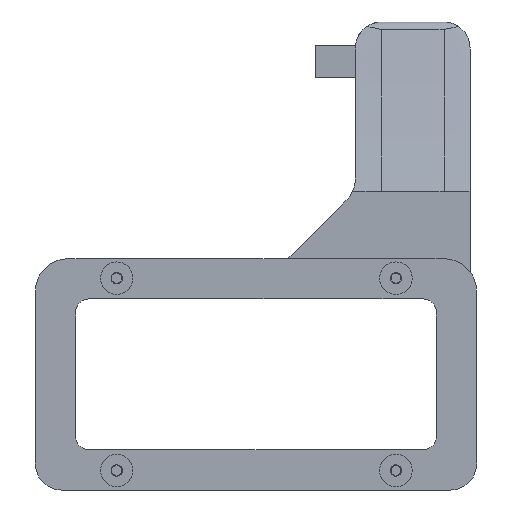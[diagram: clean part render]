
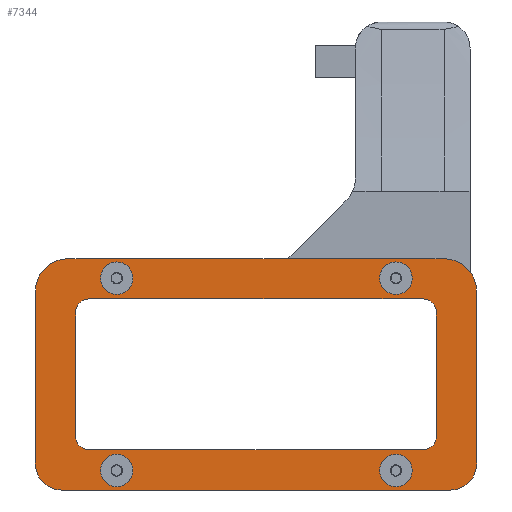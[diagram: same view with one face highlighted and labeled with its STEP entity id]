
A CAD part, front view. The second image highlights one B-rep face of the part: STEP entity #7344.
In plain terms, the highlighted planar face has unit normal (0, -1, 0).
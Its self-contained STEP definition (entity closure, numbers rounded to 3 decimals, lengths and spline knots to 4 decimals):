
#148=LINE($,#29468,#426);
#155=LINE($,#29518,#433);
#163=LINE($,#29570,#441);
#168=LINE($,#29579,#446);
#172=LINE($,#29596,#450);
#175=LINE($,#29603,#453);
#176=LINE($,#29606,#454);
#177=LINE($,#29607,#455);
#178=LINE($,#29613,#456);
#179=LINE($,#29615,#457);
#180=LINE($,#29617,#458);
#181=LINE($,#29621,#459);
#426=VECTOR($,#8607,2.6586);
#433=VECTOR($,#8652,1.9192);
#441=VECTOR($,#8702,5.1467);
#446=VECTOR($,#8709,5.986);
#450=VECTOR($,#8725,0.1144);
#453=VECTOR($,#8732,2.6586);
#454=VECTOR($,#8735,2.704);
#455=VECTOR($,#8736,2.9676);
#456=VECTOR($,#8741,2.648);
#457=VECTOR($,#8742,0.1144);
#458=VECTOR($,#8743,2.3843);
#459=VECTOR($,#8746,1.9192);
#653=FACE_BOUND($,#1912,.T.);
#654=FACE_BOUND($,#1913,.T.);
#655=FACE_BOUND($,#1914,.T.);
#656=FACE_BOUND($,#1915,.T.);
#657=FACE_BOUND($,#1916,.T.);
#757=PLANE($,#7790);
#1577=FACE_OUTER_BOUND($,#1911,.T.);
#1911=EDGE_LOOP($,(#6174,#6175,#6176,#6177,#6178,#6179,#6180,#6181,#6182,
#6183));
#1912=EDGE_LOOP($,(#6184));
#1913=EDGE_LOOP($,(#6185));
#1914=EDGE_LOOP($,(#6186));
#1915=EDGE_LOOP($,(#6187));
#1916=EDGE_LOOP($,(#6188,#6189,#6190,#6191,#6192,#6193,#6194,#6195,#6196,
#6197));
#2178=CIRCLE($,#7741,0.5);
#2189=CIRCLE($,#7758,0.2);
#2190=CIRCLE($,#7760,0.2);
#2192=CIRCLE($,#7765,0.25);
#2195=CIRCLE($,#7770,0.25);
#2196=CIRCLE($,#7772,0.4);
#2205=CIRCLE($,#7791,0.4);
#2206=CIRCLE($,#7792,0.5);
#2207=CIRCLE($,#7793,0.25);
#2208=CIRCLE($,#7794,0.25);
#2209=CIRCLE($,#7795,0.2);
#2210=CIRCLE($,#7796,0.2);
#3079=VERTEX_POINT($,#29460);
#3080=VERTEX_POINT($,#29462);
#3081=VERTEX_POINT($,#29466);
#3094=VERTEX_POINT($,#29506);
#3095=VERTEX_POINT($,#29508);
#3096=VERTEX_POINT($,#29512);
#3097=VERTEX_POINT($,#29514);
#3099=VERTEX_POINT($,#29523);
#3102=VERTEX_POINT($,#29531);
#3103=VERTEX_POINT($,#29534);
#3114=VERTEX_POINT($,#29569);
#3117=VERTEX_POINT($,#29577);
#3123=VERTEX_POINT($,#29594);
#3124=VERTEX_POINT($,#29595);
#3125=VERTEX_POINT($,#29600);
#3126=VERTEX_POINT($,#29602);
#3127=VERTEX_POINT($,#29604);
#3128=VERTEX_POINT($,#29608);
#3129=VERTEX_POINT($,#29610);
#3130=VERTEX_POINT($,#29612);
#3131=VERTEX_POINT($,#29614);
#3132=VERTEX_POINT($,#29616);
#3133=VERTEX_POINT($,#29618);
#3134=VERTEX_POINT($,#29620);
#4165=EDGE_CURVE($,#3080,#3079,#2178,.T.);
#4168=EDGE_CURVE($,#3079,#3081,#148,.T.);
#4184=EDGE_CURVE($,#3094,#3095,#2189,.T.);
#4187=EDGE_CURVE($,#3096,#3097,#2190,.T.);
#4189=EDGE_CURVE($,#3094,#3097,#155,.T.);
#4191=EDGE_CURVE($,#3099,#3099,#2192,.T.);
#4194=EDGE_CURVE($,#3102,#3102,#2195,.T.);
#4196=EDGE_CURVE($,#3081,#3103,#2196,.T.);
#4209=EDGE_CURVE($,#3114,#3095,#163,.T.);
#4214=EDGE_CURVE($,#3103,#3117,#168,.T.);
#4221=EDGE_CURVE($,#3123,#3124,#172,.T.);
#4224=EDGE_CURVE($,#3117,#3125,#2205,.T.);
#4225=EDGE_CURVE($,#3125,#3126,#175,.T.);
#4226=EDGE_CURVE($,#3126,#3127,#2206,.T.);
#4227=EDGE_CURVE($,#3127,#3123,#176,.T.);
#4228=EDGE_CURVE($,#3124,#3080,#177,.T.);
#4229=EDGE_CURVE($,#3128,#3128,#2207,.T.);
#4230=EDGE_CURVE($,#3129,#3129,#2208,.T.);
#4231=EDGE_CURVE($,#3096,#3130,#178,.T.);
#4232=EDGE_CURVE($,#3130,#3131,#179,.T.);
#4233=EDGE_CURVE($,#3131,#3132,#180,.T.);
#4234=EDGE_CURVE($,#3133,#3132,#2209,.T.);
#4235=EDGE_CURVE($,#3133,#3134,#181,.T.);
#4236=EDGE_CURVE($,#3114,#3134,#2210,.T.);
#6174=ORIENTED_EDGE($,*,*,#4214,.T.);
#6175=ORIENTED_EDGE($,*,*,#4224,.T.);
#6176=ORIENTED_EDGE($,*,*,#4225,.T.);
#6177=ORIENTED_EDGE($,*,*,#4226,.T.);
#6178=ORIENTED_EDGE($,*,*,#4227,.T.);
#6179=ORIENTED_EDGE($,*,*,#4221,.T.);
#6180=ORIENTED_EDGE($,*,*,#4228,.T.);
#6181=ORIENTED_EDGE($,*,*,#4165,.T.);
#6182=ORIENTED_EDGE($,*,*,#4168,.T.);
#6183=ORIENTED_EDGE($,*,*,#4196,.T.);
#6184=ORIENTED_EDGE($,*,*,#4191,.T.);
#6185=ORIENTED_EDGE($,*,*,#4194,.T.);
#6186=ORIENTED_EDGE($,*,*,#4229,.T.);
#6187=ORIENTED_EDGE($,*,*,#4230,.T.);
#6188=ORIENTED_EDGE($,*,*,#4209,.T.);
#6189=ORIENTED_EDGE($,*,*,#4184,.F.);
#6190=ORIENTED_EDGE($,*,*,#4189,.T.);
#6191=ORIENTED_EDGE($,*,*,#4187,.F.);
#6192=ORIENTED_EDGE($,*,*,#4231,.T.);
#6193=ORIENTED_EDGE($,*,*,#4232,.T.);
#6194=ORIENTED_EDGE($,*,*,#4233,.T.);
#6195=ORIENTED_EDGE($,*,*,#4234,.F.);
#6196=ORIENTED_EDGE($,*,*,#4235,.T.);
#6197=ORIENTED_EDGE($,*,*,#4236,.F.);
#7344=ADVANCED_FACE($,(#1577,#653,#654,#655,#656,#657),#757,.T.);
#7741=AXIS2_PLACEMENT_3D($,#29463,#8601,#8602);
#7758=AXIS2_PLACEMENT_3D($,#29509,#8641,#8642);
#7760=AXIS2_PLACEMENT_3D($,#29515,#8647,#8648);
#7765=AXIS2_PLACEMENT_3D($,#29524,#8659,#8660);
#7770=AXIS2_PLACEMENT_3D($,#29532,#8669,#8670);
#7772=AXIS2_PLACEMENT_3D($,#29536,#8674,#8675);
#7790=AXIS2_PLACEMENT_3D($,#29599,#8728,#8729);
#7791=AXIS2_PLACEMENT_3D($,#29601,#8730,#8731);
#7792=AXIS2_PLACEMENT_3D($,#29605,#8733,#8734);
#7793=AXIS2_PLACEMENT_3D($,#29609,#8737,#8738);
#7794=AXIS2_PLACEMENT_3D($,#29611,#8739,#8740);
#7795=AXIS2_PLACEMENT_3D($,#29619,#8744,#8745);
#7796=AXIS2_PLACEMENT_3D($,#29622,#8747,#8748);
#8601=DIRECTION('center_axis',(0.,-1.,0.));
#8602=DIRECTION('ref_axis',(0.,0.,1.));
#8607=DIRECTION($,(0.,0.,-1.));
#8641=DIRECTION('center_axis',(0.,-1.,0.));
#8642=DIRECTION('ref_axis',(-0.707,0.,-0.707));
#8647=DIRECTION('center_axis',(0.,-1.,0.));
#8648=DIRECTION('ref_axis',(-0.707,0.,0.707));
#8652=DIRECTION($,(0.,0.,1.));
#8659=DIRECTION('center_axis',(0.,1.,0.));
#8660=DIRECTION('ref_axis',(0.,0.,-1.));
#8669=DIRECTION('center_axis',(0.,1.,0.));
#8670=DIRECTION('ref_axis',(0.,0.,-1.));
#8674=DIRECTION('center_axis',(0.,-1.,0.));
#8675=DIRECTION('ref_axis',(-1.,0.,0.));
#8702=DIRECTION($,(-1.,0.,0.));
#8709=DIRECTION($,(1.,0.,0.));
#8725=DIRECTION($,(-1.,0.,0.));
#8728=DIRECTION('center_axis',(0.,-1.,0.));
#8729=DIRECTION('ref_axis',(1.,0.,0.));
#8730=DIRECTION('center_axis',(0.,-1.,0.));
#8731=DIRECTION('ref_axis',(0.,0.,-1.));
#8732=DIRECTION($,(0.,0.,1.));
#8733=DIRECTION('center_axis',(0.,-1.,0.));
#8734=DIRECTION('ref_axis',(1.,0.,0.));
#8735=DIRECTION($,(-1.,0.,0.));
#8736=DIRECTION($,(-1.,0.,0.));
#8737=DIRECTION('center_axis',(0.,1.,0.));
#8738=DIRECTION('ref_axis',(0.,0.,-1.));
#8739=DIRECTION('center_axis',(0.,1.,0.));
#8740=DIRECTION('ref_axis',(0.,0.,-1.));
#8741=DIRECTION($,(1.,0.,0.));
#8742=DIRECTION($,(1.,0.,0.));
#8743=DIRECTION($,(1.,0.,0.));
#8744=DIRECTION('center_axis',(0.,-1.,0.));
#8745=DIRECTION('ref_axis',(0.707,0.,0.707));
#8746=DIRECTION($,(0.,0.,-1.));
#8747=DIRECTION('center_axis',(0.,-1.,0.));
#8748=DIRECTION('ref_axis',(0.707,0.,-0.707));
#29460=CARTESIAN_POINT('',(12.0904,8.0209,19.7919));
#29462=CARTESIAN_POINT('',(12.5904,8.0209,20.2919));
#29463=CARTESIAN_POINT('Origin',(12.5904,8.0209,19.7919));
#29466=CARTESIAN_POINT('',(12.0904,8.0209,17.1334));
#29468=CARTESIAN_POINT($,(12.0904,8.0209,19.7919));
#29506=CARTESIAN_POINT('',(12.7101,8.0209,17.553));
#29508=CARTESIAN_POINT('',(12.9101,8.0209,17.353));
#29509=CARTESIAN_POINT('Origin',(12.9101,8.0209,17.553));
#29512=CARTESIAN_POINT('',(12.9101,8.0209,19.6723));
#29514=CARTESIAN_POINT('',(12.7101,8.0209,19.4723));
#29515=CARTESIAN_POINT('Origin',(12.9101,8.0209,19.4723));
#29518=CARTESIAN_POINT($,(12.7101,8.0209,17.9328));
#29523=CARTESIAN_POINT('',(13.3404,8.0209,17.2834));
#29524=CARTESIAN_POINT('Origin',(13.3404,8.0209,17.0334));
#29531=CARTESIAN_POINT('',(13.3404,8.0209,20.2419));
#29532=CARTESIAN_POINT('Origin',(13.3404,8.0209,19.9919));
#29534=CARTESIAN_POINT('',(12.4904,8.0209,16.7334));
#29536=CARTESIAN_POINT('Origin',(12.4904,8.0209,17.1334));
#29569=CARTESIAN_POINT('',(18.0568,8.0209,17.353));
#29570=CARTESIAN_POINT($,(16.7951,8.0209,17.353));
#29577=CARTESIAN_POINT('',(18.4764,8.0209,16.7334));
#29579=CARTESIAN_POINT($,(12.1904,8.0209,16.7334));
#29594=CARTESIAN_POINT('',(15.6724,8.0209,20.2919));
#29595=CARTESIAN_POINT('',(15.5581,8.0209,20.2919));
#29596=CARTESIAN_POINT($,(15.6724,8.0209,20.2919));
#29599=CARTESIAN_POINT('Origin',(15.3334,8.0209,18.5126));
#29600=CARTESIAN_POINT('',(18.8764,8.0209,17.1334));
#29601=CARTESIAN_POINT('Origin',(18.4764,8.0209,17.1334));
#29602=CARTESIAN_POINT('',(18.8764,8.0209,19.7919));
#29603=CARTESIAN_POINT($,(18.8764,8.0209,17.1334));
#29604=CARTESIAN_POINT('',(18.3764,8.0209,20.2919));
#29605=CARTESIAN_POINT('Origin',(18.3764,8.0209,19.7919));
#29606=CARTESIAN_POINT($,(18.3764,8.0209,20.2919));
#29607=CARTESIAN_POINT($,(15.8581,8.0209,20.2919));
#29608=CARTESIAN_POINT('',(17.6364,8.0209,20.2419));
#29609=CARTESIAN_POINT('Origin',(17.6364,8.0209,19.9919));
#29610=CARTESIAN_POINT('',(17.6364,8.0209,17.2834));
#29611=CARTESIAN_POINT('Origin',(17.6364,8.0209,17.0334));
#29612=CARTESIAN_POINT('',(15.5581,8.0209,19.6723));
#29613=CARTESIAN_POINT($,(13.8718,8.0209,19.6723));
#29614=CARTESIAN_POINT('',(15.6725,8.0209,19.6723));
#29615=CARTESIAN_POINT($,(15.4458,8.0209,19.6723));
#29616=CARTESIAN_POINT('',(18.0568,8.0209,19.6723));
#29617=CARTESIAN_POINT($,(15.5029,8.0209,19.6723));
#29618=CARTESIAN_POINT('',(18.2568,8.0209,19.4723));
#29619=CARTESIAN_POINT('Origin',(18.0568,8.0209,19.4723));
#29620=CARTESIAN_POINT('',(18.2568,8.0209,17.553));
#29621=CARTESIAN_POINT($,(18.2568,8.0209,19.0924));
#29622=CARTESIAN_POINT('Origin',(18.0568,8.0209,17.553));
